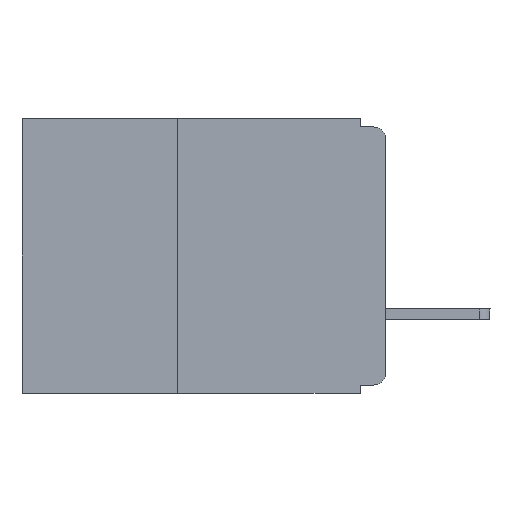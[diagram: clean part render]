
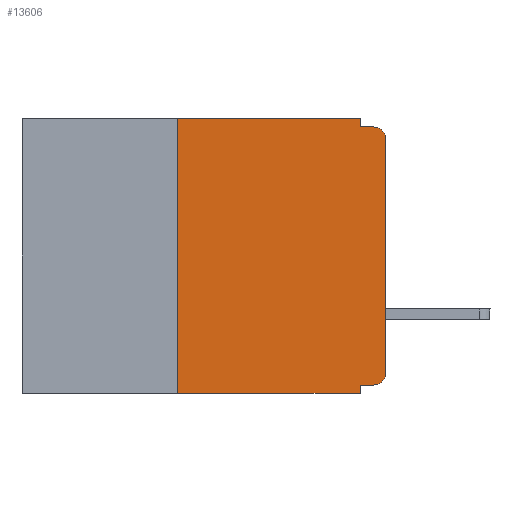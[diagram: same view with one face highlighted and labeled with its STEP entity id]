
A CAD part, left-side view. The second image highlights one B-rep face of the part: STEP entity #13606.
In plain terms, the highlighted planar face has unit normal (-1, 0, 0).
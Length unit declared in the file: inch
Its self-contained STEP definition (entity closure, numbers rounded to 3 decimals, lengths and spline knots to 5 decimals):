
#78 = DIRECTION ( 'NONE',  ( 0., 0., 1. ) ) ;
#245 = LINE ( 'NONE', #14185, #652 ) ;
#614 = ORIENTED_EDGE ( 'NONE', *, *, #12682, .F. ) ;
#652 = VECTOR ( 'NONE', #6295, 39.37008 ) ;
#701 = CARTESIAN_POINT ( 'NONE',  ( 0., 0.031, -0.01 ) ) ;
#1010 = VERTEX_POINT ( 'NONE', #2741 ) ;
#1087 = VECTOR ( 'NONE', #9378, 39.37008 ) ;
#1291 = CARTESIAN_POINT ( 'NONE',  ( 0., 0.437, 0. ) ) ;
#1455 = VECTOR ( 'NONE', #7843, 39.37008 ) ;
#1547 = ORIENTED_EDGE ( 'NONE', *, *, #15355, .T. ) ;
#2221 = CARTESIAN_POINT ( 'NONE',  ( 0., 0.015, -0.305 ) ) ;
#2713 = LINE ( 'NONE', #14295, #1455 ) ;
#2741 = CARTESIAN_POINT ( 'NONE',  ( 0., 0.031, -0.32 ) ) ;
#3271 = EDGE_CURVE ( 'NONE', #1010, #10531, #16555, .T. ) ;
#3754 = CARTESIAN_POINT ( 'NONE',  ( 0., 0.25, 0. ) ) ;
#3995 = LINE ( 'NONE', #12088, #10205 ) ;
#4282 = VERTEX_POINT ( 'NONE', #9158 ) ;
#4571 = VERTEX_POINT ( 'NONE', #3754 ) ;
#5071 = DIRECTION ( 'NONE',  ( 1., 0., 0. ) ) ;
#5340 = VECTOR ( 'NONE', #17183, 39.37008 ) ;
#5768 = VERTEX_POINT ( 'NONE', #701 ) ;
#5774 = CARTESIAN_POINT ( 'NONE',  ( 0., 0., -0.025 ) ) ;
#6144 = VECTOR ( 'NONE', #16327, 39.37008 ) ;
#6256 = DIRECTION ( 'NONE',  ( 0., 0., -1. ) ) ;
#6295 = DIRECTION ( 'NONE',  ( 0., 0., -1. ) ) ;
#6383 = VERTEX_POINT ( 'NONE', #9648 ) ;
#7246 = CARTESIAN_POINT ( 'NONE',  ( 0., 0.015, -0.025 ) ) ;
#7749 = ORIENTED_EDGE ( 'NONE', *, *, #11208, .F. ) ;
#7843 = DIRECTION ( 'NONE',  ( 0., -1., 0. ) ) ;
#7994 = CARTESIAN_POINT ( 'NONE',  ( 0., 0.437, 0. ) ) ;
#8151 = LINE ( 'NONE', #16029, #1087 ) ;
#8613 = DIRECTION ( 'NONE',  ( 0., 1., 0. ) ) ;
#8804 = ORIENTED_EDGE ( 'NONE', *, *, #9771, .T. ) ;
#8914 = ORIENTED_EDGE ( 'NONE', *, *, #3271, .F. ) ;
#9069 = PLANE ( 'NONE',  #10971 ) ;
#9115 = VERTEX_POINT ( 'NONE', #14103 ) ;
#9158 = CARTESIAN_POINT ( 'NONE',  ( 0., 0.031, 0. ) ) ;
#9178 = DIRECTION ( 'NONE',  ( 0., 0., -1. ) ) ;
#9253 = FACE_OUTER_BOUND ( 'NONE', #16257, .T. ) ;
#9378 = DIRECTION ( 'NONE',  ( 0., -1., 0. ) ) ;
#9416 = EDGE_CURVE ( 'NONE', #12187, #13836, #11069, .T. ) ;
#9534 = LINE ( 'NONE', #9849, #15789 ) ;
#9648 = CARTESIAN_POINT ( 'NONE',  ( 0., 0.015, -0.32 ) ) ;
#9771 = EDGE_CURVE ( 'NONE', #13533, #10531, #8151, .T. ) ;
#9849 = CARTESIAN_POINT ( 'NONE',  ( 0., 0., -0.32 ) ) ;
#10016 = CARTESIAN_POINT ( 'NONE',  ( 0., 0.015, -0.01 ) ) ;
#10023 = EDGE_CURVE ( 'NONE', #4282, #5768, #245, .T. ) ;
#10077 = DIRECTION ( 'NONE',  ( 0., 0., -1. ) ) ;
#10205 = VECTOR ( 'NONE', #78, 39.37008 ) ;
#10376 = DIRECTION ( 'NONE',  ( -1., 0., 0. ) ) ;
#10531 = VERTEX_POINT ( 'NONE', #16790 ) ;
#10576 = CARTESIAN_POINT ( 'NONE',  ( 0., 0.25, -0.33 ) ) ;
#10971 = AXIS2_PLACEMENT_3D ( 'NONE', #1291, #5071, #9178 ) ;
#11068 = EDGE_CURVE ( 'NONE', #6383, #1010, #9534, .T. ) ;
#11069 = CIRCLE ( 'NONE', #11801, 0.015 ) ;
#11074 = CARTESIAN_POINT ( 'NONE',  ( 0., 0.031, -0.33 ) ) ;
#11208 = EDGE_CURVE ( 'NONE', #13533, #4571, #16613, .T. ) ;
#11735 = CIRCLE ( 'NONE', #14955, 0.015 ) ;
#11801 = AXIS2_PLACEMENT_3D ( 'NONE', #7246, #10376, #6256 ) ;
#12088 = CARTESIAN_POINT ( 'NONE',  ( 0., 0., 0. ) ) ;
#12102 = ORIENTED_EDGE ( 'NONE', *, *, #12869, .T. ) ;
#12162 = VECTOR ( 'NONE', #13339, 39.37008 ) ;
#12187 = VERTEX_POINT ( 'NONE', #5774 ) ;
#12473 = ORIENTED_EDGE ( 'NONE', *, *, #10023, .F. ) ;
#12682 = EDGE_CURVE ( 'NONE', #4571, #4282, #16339, .T. ) ;
#12869 = EDGE_CURVE ( 'NONE', #6383, #9115, #11735, .T. ) ;
#13339 = DIRECTION ( 'NONE',  ( 0., -1., 0. ) ) ;
#13533 = VERTEX_POINT ( 'NONE', #10576 ) ;
#13606 = ADVANCED_FACE ( 'NONE', ( #9253 ), #9069, .F. ) ;
#13836 = VERTEX_POINT ( 'NONE', #10016 ) ;
#14103 = CARTESIAN_POINT ( 'NONE',  ( 0., 0., -0.305 ) ) ;
#14185 = CARTESIAN_POINT ( 'NONE',  ( 0., 0.031, 0. ) ) ;
#14295 = CARTESIAN_POINT ( 'NONE',  ( 0., 0., -0.01 ) ) ;
#14311 = ORIENTED_EDGE ( 'NONE', *, *, #9416, .T. ) ;
#14320 = DIRECTION ( 'NONE',  ( -1., 0., 0. ) ) ;
#14503 = CARTESIAN_POINT ( 'NONE',  ( 0., 0.25, -0.33 ) ) ;
#14955 = AXIS2_PLACEMENT_3D ( 'NONE', #2221, #14320, #10077 ) ;
#15355 = EDGE_CURVE ( 'NONE', #9115, #12187, #3995, .T. ) ;
#15576 = ORIENTED_EDGE ( 'NONE', *, *, #16437, .F. ) ;
#15789 = VECTOR ( 'NONE', #8613, 39.37008 ) ;
#16029 = CARTESIAN_POINT ( 'NONE',  ( 0., 0.437, -0.33 ) ) ;
#16257 = EDGE_LOOP ( 'NONE', ( #1547, #14311, #15576, #12473, #614, #7749, #8804, #8914, #16955, #12102 ) ) ;
#16327 = DIRECTION ( 'NONE',  ( 0., 0., -1. ) ) ;
#16339 = LINE ( 'NONE', #7994, #12162 ) ;
#16437 = EDGE_CURVE ( 'NONE', #5768, #13836, #2713, .T. ) ;
#16555 = LINE ( 'NONE', #11074, #6144 ) ;
#16613 = LINE ( 'NONE', #14503, #5340 ) ;
#16790 = CARTESIAN_POINT ( 'NONE',  ( 0., 0.031, -0.33 ) ) ;
#16955 = ORIENTED_EDGE ( 'NONE', *, *, #11068, .F. ) ;
#17183 = DIRECTION ( 'NONE',  ( 0., 0., 1. ) ) ;
